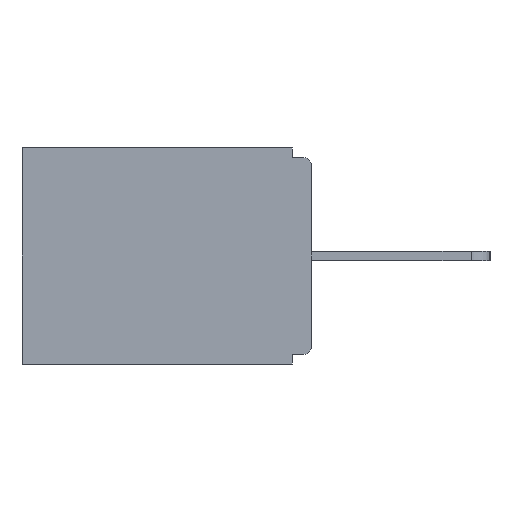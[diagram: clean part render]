
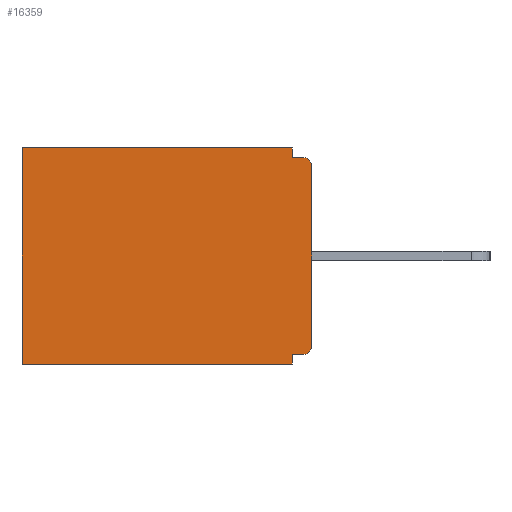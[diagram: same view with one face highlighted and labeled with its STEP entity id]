
A CAD part, left-side view. The second image highlights one B-rep face of the part: STEP entity #16359.
In plain terms, the highlighted planar face has unit normal (-1, 0, 0).
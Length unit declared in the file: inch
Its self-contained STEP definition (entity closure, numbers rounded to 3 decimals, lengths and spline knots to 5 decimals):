
#120 = LINE ( 'NONE', #13794, #16324 ) ;
#291 = LINE ( 'NONE', #13917, #16461 ) ;
#431 = ORIENTED_EDGE ( 'NONE', *, *, #12768, .F. ) ;
#648 = EDGE_CURVE ( 'NONE', #12201, #7025, #120, .T. ) ;
#865 = ORIENTED_EDGE ( 'NONE', *, *, #10458, .T. ) ;
#1058 = PLANE ( 'NONE',  #6087 ) ;
#1571 = EDGE_CURVE ( 'NONE', #7025, #8207, #15933, .T. ) ;
#1960 = DIRECTION ( 'NONE',  ( 0., 1., 0. ) ) ;
#2030 = EDGE_LOOP ( 'NONE', ( #865, #5282, #13277, #5296, #16389, #9582, #8408, #13093, #7831, #431 ) ) ;
#2462 = DIRECTION ( 'NONE',  ( 0., 0., -1. ) ) ;
#2742 = VERTEX_POINT ( 'NONE', #10270 ) ;
#2759 = VERTEX_POINT ( 'NONE', #11993 ) ;
#2915 = VECTOR ( 'NONE', #9535, 39.37008 ) ;
#4250 = CARTESIAN_POINT ( 'NONE',  ( 0.298, 0.46, 0. ) ) ;
#4261 = CARTESIAN_POINT ( 'NONE',  ( 0.298, 0.031, -0.328 ) ) ;
#4540 = DIRECTION ( 'NONE',  ( 0., -1., 0. ) ) ;
#4776 = CIRCLE ( 'NONE', #12215, 0.015 ) ;
#5037 = CARTESIAN_POINT ( 'NONE',  ( 0.298, 0.031, -0.343 ) ) ;
#5282 = ORIENTED_EDGE ( 'NONE', *, *, #12838, .F. ) ;
#5296 = ORIENTED_EDGE ( 'NONE', *, *, #10521, .T. ) ;
#5425 = VECTOR ( 'NONE', #4540, 39.37008 ) ;
#6087 = AXIS2_PLACEMENT_3D ( 'NONE', #16271, #10236, #2462 ) ;
#6236 = CARTESIAN_POINT ( 'NONE',  ( 0.298, 0., -0.343 ) ) ;
#6791 = LINE ( 'NONE', #5037, #13858 ) ;
#7025 = VERTEX_POINT ( 'NONE', #7128 ) ;
#7128 = CARTESIAN_POINT ( 'NONE',  ( 0.298, 0.031, -0.343 ) ) ;
#7194 = EDGE_CURVE ( 'NONE', #8455, #8207, #10287, .T. ) ;
#7287 = VECTOR ( 'NONE', #8906, 39.37008 ) ;
#7413 = VERTEX_POINT ( 'NONE', #11590 ) ;
#7548 = DIRECTION ( 'NONE',  ( -1., 0., 0. ) ) ;
#7563 = CARTESIAN_POINT ( 'NONE',  ( 0.298, 0.015, -0.313 ) ) ;
#7599 = CARTESIAN_POINT ( 'NONE',  ( 0.298, 0.031, -0.015 ) ) ;
#7645 = DIRECTION ( 'NONE',  ( 0., 0., -1. ) ) ;
#7831 = ORIENTED_EDGE ( 'NONE', *, *, #10791, .T. ) ;
#8207 = VERTEX_POINT ( 'NONE', #12043 ) ;
#8231 = DIRECTION ( 'NONE',  ( 0., 0., -1. ) ) ;
#8408 = ORIENTED_EDGE ( 'NONE', *, *, #648, .F. ) ;
#8455 = VERTEX_POINT ( 'NONE', #4250 ) ;
#8886 = FACE_OUTER_BOUND ( 'NONE', #2030, .T. ) ;
#8906 = DIRECTION ( 'NONE',  ( 0., 0., -1. ) ) ;
#9054 = DIRECTION ( 'NONE',  ( 0., 0., -1. ) ) ;
#9535 = DIRECTION ( 'NONE',  ( 0., 1., 0. ) ) ;
#9582 = ORIENTED_EDGE ( 'NONE', *, *, #1571, .F. ) ;
#9643 = LINE ( 'NONE', #14429, #12603 ) ;
#9645 = CARTESIAN_POINT ( 'NONE',  ( 0.298, 0.46, 0. ) ) ;
#10228 = LINE ( 'NONE', #15744, #2915 ) ;
#10236 = DIRECTION ( 'NONE',  ( 1., 0., 0. ) ) ;
#10270 = CARTESIAN_POINT ( 'NONE',  ( 0.298, 0., -0.313 ) ) ;
#10287 = LINE ( 'NONE', #9645, #7287 ) ;
#10458 = EDGE_CURVE ( 'NONE', #11976, #2759, #4776, .T. ) ;
#10521 = EDGE_CURVE ( 'NONE', #12876, #8455, #291, .T. ) ;
#10619 = VERTEX_POINT ( 'NONE', #7599 ) ;
#10791 = EDGE_CURVE ( 'NONE', #7413, #2742, #13096, .T. ) ;
#11590 = CARTESIAN_POINT ( 'NONE',  ( 0.298, 0.015, -0.328 ) ) ;
#11851 = LINE ( 'NONE', #15807, #5425 ) ;
#11976 = VERTEX_POINT ( 'NONE', #13870 ) ;
#11993 = CARTESIAN_POINT ( 'NONE',  ( 0.298, 0.015, -0.015 ) ) ;
#12043 = CARTESIAN_POINT ( 'NONE',  ( 0.298, 0.46, -0.343 ) ) ;
#12201 = VERTEX_POINT ( 'NONE', #4261 ) ;
#12215 = AXIS2_PLACEMENT_3D ( 'NONE', #15702, #14551, #14532 ) ;
#12603 = VECTOR ( 'NONE', #8231, 39.37008 ) ;
#12768 = EDGE_CURVE ( 'NONE', #11976, #2742, #9643, .T. ) ;
#12838 = EDGE_CURVE ( 'NONE', #10619, #2759, #11851, .T. ) ;
#12876 = VERTEX_POINT ( 'NONE', #14638 ) ;
#13093 = ORIENTED_EDGE ( 'NONE', *, *, #13388, .F. ) ;
#13096 = CIRCLE ( 'NONE', #14332, 0.015 ) ;
#13114 = VECTOR ( 'NONE', #1960, 39.37008 ) ;
#13130 = DIRECTION ( 'NONE',  ( 0., 1., 0. ) ) ;
#13277 = ORIENTED_EDGE ( 'NONE', *, *, #14258, .F. ) ;
#13388 = EDGE_CURVE ( 'NONE', #7413, #12201, #10228, .T. ) ;
#13794 = CARTESIAN_POINT ( 'NONE',  ( 0.298, 0.031, -0.343 ) ) ;
#13854 = DIRECTION ( 'NONE',  ( 0., 0., -1. ) ) ;
#13858 = VECTOR ( 'NONE', #13854, 39.37008 ) ;
#13870 = CARTESIAN_POINT ( 'NONE',  ( 0.298, 0., -0.03 ) ) ;
#13917 = CARTESIAN_POINT ( 'NONE',  ( 0.298, 0., 0. ) ) ;
#14258 = EDGE_CURVE ( 'NONE', #12876, #10619, #6791, .T. ) ;
#14332 = AXIS2_PLACEMENT_3D ( 'NONE', #7563, #7548, #7645 ) ;
#14429 = CARTESIAN_POINT ( 'NONE',  ( 0.298, 0., 0. ) ) ;
#14532 = DIRECTION ( 'NONE',  ( 0., 0., -1. ) ) ;
#14551 = DIRECTION ( 'NONE',  ( -1., 0., 0. ) ) ;
#14638 = CARTESIAN_POINT ( 'NONE',  ( 0.298, 0.031, 0. ) ) ;
#15702 = CARTESIAN_POINT ( 'NONE',  ( 0.298, 0.015, -0.03 ) ) ;
#15744 = CARTESIAN_POINT ( 'NONE',  ( 0.298, 0., -0.328 ) ) ;
#15807 = CARTESIAN_POINT ( 'NONE',  ( 0.298, 0., -0.015 ) ) ;
#15933 = LINE ( 'NONE', #6236, #13114 ) ;
#16271 = CARTESIAN_POINT ( 'NONE',  ( 0.298, 0., 0. ) ) ;
#16324 = VECTOR ( 'NONE', #9054, 39.37008 ) ;
#16359 = ADVANCED_FACE ( 'NONE', ( #8886 ), #1058, .F. ) ;
#16389 = ORIENTED_EDGE ( 'NONE', *, *, #7194, .T. ) ;
#16461 = VECTOR ( 'NONE', #13130, 39.37008 ) ;
